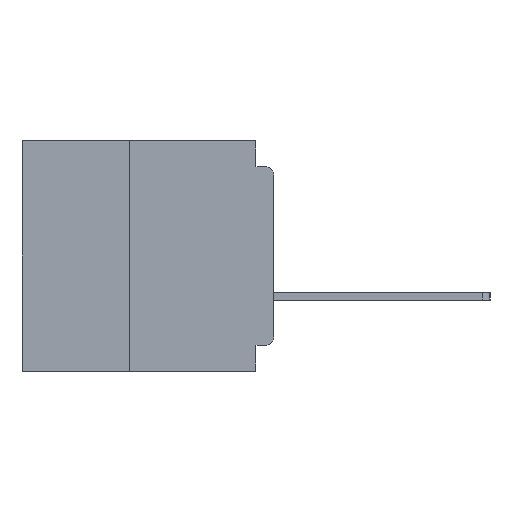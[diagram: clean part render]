
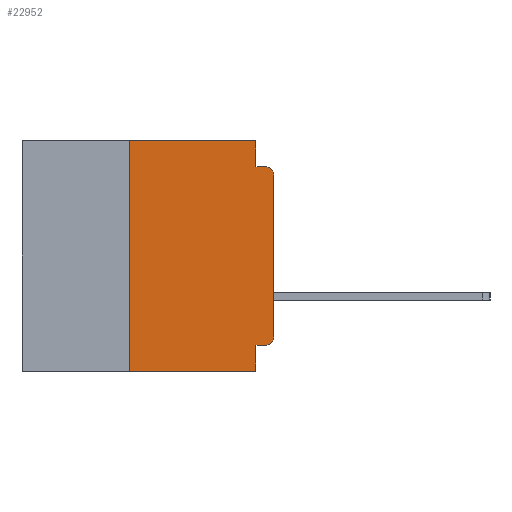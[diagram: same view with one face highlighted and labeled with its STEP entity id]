
A CAD part, left-side view. The second image highlights one B-rep face of the part: STEP entity #22952.
In plain terms, the highlighted planar face has unit normal (-1, 0, 0).
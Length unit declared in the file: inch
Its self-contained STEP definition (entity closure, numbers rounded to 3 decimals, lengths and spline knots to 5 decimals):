
#633 = DIRECTION ( 'NONE',  ( -1., 0., 0. ) ) ;
#1055 = PLANE ( 'NONE',  #12733 ) ;
#1439 = ORIENTED_EDGE ( 'NONE', *, *, #60058, .F. ) ;
#2142 = VECTOR ( 'NONE', #61757, 39.37008 ) ;
#2164 = EDGE_LOOP ( 'NONE', ( #47524, #24245, #3868, #58365, #26486, #1439, #19483, #25746, #53705, #20303 ) ) ;
#2577 = LINE ( 'NONE', #6501, #11163 ) ;
#3797 = DIRECTION ( 'NONE',  ( -1., 0., 0. ) ) ;
#3851 = CARTESIAN_POINT ( 'NONE',  ( 0., 0.25, 0. ) ) ;
#3868 = ORIENTED_EDGE ( 'NONE', *, *, #23317, .F. ) ;
#4638 = VERTEX_POINT ( 'NONE', #60036 ) ;
#6501 = CARTESIAN_POINT ( 'NONE',  ( 0., 0., 0. ) ) ;
#8200 = CARTESIAN_POINT ( 'NONE',  ( 0., 0.25, -0.4 ) ) ;
#8930 = AXIS2_PLACEMENT_3D ( 'NONE', #33770, #3797, #38785 ) ;
#9109 = EDGE_CURVE ( 'NONE', #4638, #20797, #42343, .T. ) ;
#9893 = CARTESIAN_POINT ( 'NONE',  ( 0., 0.031, -0.4 ) ) ;
#10052 = VERTEX_POINT ( 'NONE', #12434 ) ;
#11163 = VECTOR ( 'NONE', #11316, 39.37008 ) ;
#11223 = CARTESIAN_POINT ( 'NONE',  ( 0., 0., -0.06 ) ) ;
#11316 = DIRECTION ( 'NONE',  ( 0., 0., 1. ) ) ;
#11334 = CARTESIAN_POINT ( 'NONE',  ( 0., 0.437, 0. ) ) ;
#12000 = CARTESIAN_POINT ( 'NONE',  ( 0., 0., -0.34 ) ) ;
#12434 = CARTESIAN_POINT ( 'NONE',  ( 0., 0.031, -0.045 ) ) ;
#12733 = AXIS2_PLACEMENT_3D ( 'NONE', #40815, #16199, #50966 ) ;
#12994 = VERTEX_POINT ( 'NONE', #15821 ) ;
#14086 = EDGE_CURVE ( 'NONE', #20416, #20797, #30447, .T. ) ;
#15137 = VERTEX_POINT ( 'NONE', #3851 ) ;
#15821 = CARTESIAN_POINT ( 'NONE',  ( 0., 0.015, -0.355 ) ) ;
#15867 = VECTOR ( 'NONE', #49763, 39.37008 ) ;
#16199 = DIRECTION ( 'NONE',  ( 1., 0., 0. ) ) ;
#18991 = CARTESIAN_POINT ( 'NONE',  ( 0., 0., -0.045 ) ) ;
#19003 = AXIS2_PLACEMENT_3D ( 'NONE', #30613, #633, #35623 ) ;
#19483 = ORIENTED_EDGE ( 'NONE', *, *, #14086, .T. ) ;
#19944 = EDGE_CURVE ( 'NONE', #49217, #10052, #40431, .T. ) ;
#20303 = ORIENTED_EDGE ( 'NONE', *, *, #23910, .T. ) ;
#20416 = VERTEX_POINT ( 'NONE', #40747 ) ;
#20630 = DIRECTION ( 'NONE',  ( 0., -1., 0. ) ) ;
#20797 = VERTEX_POINT ( 'NONE', #63594 ) ;
#22952 = ADVANCED_FACE ( 'NONE', ( #50042 ), #1055, .F. ) ;
#23079 = VERTEX_POINT ( 'NONE', #12000 ) ;
#23317 = EDGE_CURVE ( 'NONE', #10052, #59774, #28287, .T. ) ;
#23910 = EDGE_CURVE ( 'NONE', #12994, #23079, #55319, .T. ) ;
#24245 = ORIENTED_EDGE ( 'NONE', *, *, #63754, .T. ) ;
#24376 = LINE ( 'NONE', #8200, #49210 ) ;
#25746 = ORIENTED_EDGE ( 'NONE', *, *, #9109, .F. ) ;
#25898 = LINE ( 'NONE', #39456, #50739 ) ;
#26486 = ORIENTED_EDGE ( 'NONE', *, *, #33612, .F. ) ;
#27098 = CARTESIAN_POINT ( 'NONE',  ( 0., 0.031, 0. ) ) ;
#28287 = LINE ( 'NONE', #18991, #38422 ) ;
#30447 = LINE ( 'NONE', #55344, #42085 ) ;
#30490 = EDGE_CURVE ( 'NONE', #23079, #42333, #2577, .T. ) ;
#30613 = CARTESIAN_POINT ( 'NONE',  ( 0., 0.015, -0.06 ) ) ;
#31066 = VECTOR ( 'NONE', #46412, 39.37008 ) ;
#33612 = EDGE_CURVE ( 'NONE', #15137, #49217, #45813, .T. ) ;
#33770 = CARTESIAN_POINT ( 'NONE',  ( 0., 0.015, -0.34 ) ) ;
#35623 = DIRECTION ( 'NONE',  ( 0., 0., -1. ) ) ;
#36312 = CIRCLE ( 'NONE', #19003, 0.015 ) ;
#38191 = DIRECTION ( 'NONE',  ( 0., 0., 1. ) ) ;
#38422 = VECTOR ( 'NONE', #48762, 39.37008 ) ;
#38785 = DIRECTION ( 'NONE',  ( 0., 0., -1. ) ) ;
#39456 = CARTESIAN_POINT ( 'NONE',  ( 0., 0., -0.355 ) ) ;
#40028 = CARTESIAN_POINT ( 'NONE',  ( 0., 0.031, 0. ) ) ;
#40431 = LINE ( 'NONE', #27098, #2142 ) ;
#40747 = CARTESIAN_POINT ( 'NONE',  ( 0., 0.25, -0.4 ) ) ;
#40815 = CARTESIAN_POINT ( 'NONE',  ( 0., 0.437, 0. ) ) ;
#42085 = VECTOR ( 'NONE', #20630, 39.37008 ) ;
#42333 = VERTEX_POINT ( 'NONE', #11223 ) ;
#42343 = LINE ( 'NONE', #9893, #15867 ) ;
#43884 = EDGE_CURVE ( 'NONE', #12994, #4638, #25898, .T. ) ;
#44401 = DIRECTION ( 'NONE',  ( 0., 1., 0. ) ) ;
#45813 = LINE ( 'NONE', #11334, #31066 ) ;
#46412 = DIRECTION ( 'NONE',  ( 0., -1., 0. ) ) ;
#47524 = ORIENTED_EDGE ( 'NONE', *, *, #30490, .T. ) ;
#48762 = DIRECTION ( 'NONE',  ( 0., -1., 0. ) ) ;
#49210 = VECTOR ( 'NONE', #38191, 39.37008 ) ;
#49217 = VERTEX_POINT ( 'NONE', #40028 ) ;
#49763 = DIRECTION ( 'NONE',  ( 0., 0., -1. ) ) ;
#50042 = FACE_OUTER_BOUND ( 'NONE', #2164, .T. ) ;
#50739 = VECTOR ( 'NONE', #44401, 39.37008 ) ;
#50966 = DIRECTION ( 'NONE',  ( 0., 0., -1. ) ) ;
#53705 = ORIENTED_EDGE ( 'NONE', *, *, #43884, .F. ) ;
#55319 = CIRCLE ( 'NONE', #8930, 0.015 ) ;
#55344 = CARTESIAN_POINT ( 'NONE',  ( 0., 0.437, -0.4 ) ) ;
#55484 = CARTESIAN_POINT ( 'NONE',  ( 0., 0.015, -0.045 ) ) ;
#58365 = ORIENTED_EDGE ( 'NONE', *, *, #19944, .F. ) ;
#59774 = VERTEX_POINT ( 'NONE', #55484 ) ;
#60036 = CARTESIAN_POINT ( 'NONE',  ( 0., 0.031, -0.355 ) ) ;
#60058 = EDGE_CURVE ( 'NONE', #20416, #15137, #24376, .T. ) ;
#61757 = DIRECTION ( 'NONE',  ( 0., 0., -1. ) ) ;
#63594 = CARTESIAN_POINT ( 'NONE',  ( 0., 0.031, -0.4 ) ) ;
#63754 = EDGE_CURVE ( 'NONE', #42333, #59774, #36312, .T. ) ;
